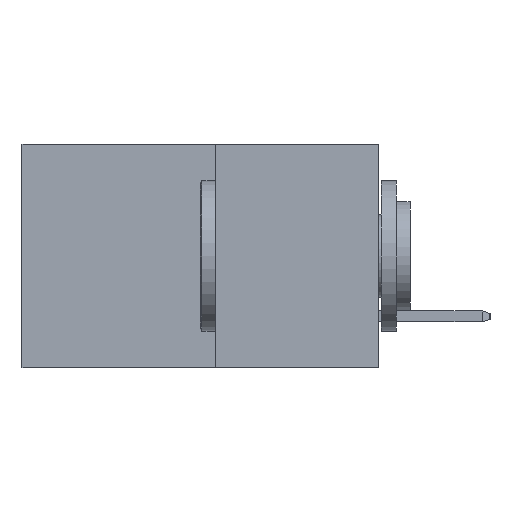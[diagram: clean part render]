
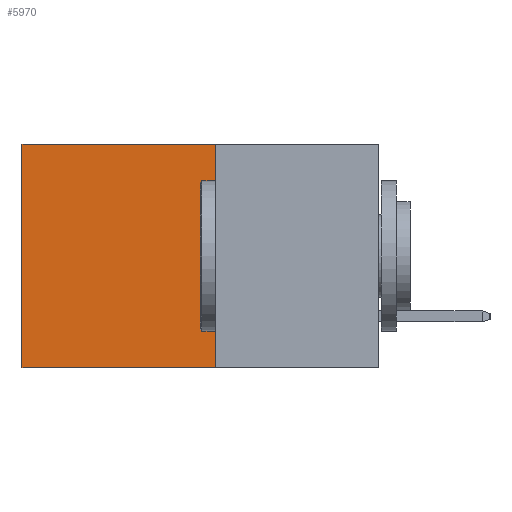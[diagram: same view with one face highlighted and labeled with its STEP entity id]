
A CAD part, left-side view. The second image highlights one B-rep face of the part: STEP entity #5970.
In plain terms, the highlighted planar face has unit normal (-1, 0, 0).
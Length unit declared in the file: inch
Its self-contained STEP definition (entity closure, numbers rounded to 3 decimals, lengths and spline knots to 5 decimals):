
#298 = VERTEX_POINT ( 'NONE', #609 ) ;
#563 = VERTEX_POINT ( 'NONE', #2316 ) ;
#609 = CARTESIAN_POINT ( 'NONE',  ( 0.277, 0.59, -0.37 ) ) ;
#874 = EDGE_CURVE ( 'NONE', #563, #6993, #4455, .T. ) ;
#967 = DIRECTION ( 'NONE',  ( 0., 0., -1. ) ) ;
#1221 = DIRECTION ( 'NONE',  ( 0., 0., -1. ) ) ;
#1283 = DIRECTION ( 'NONE',  ( 1., 0., 0. ) ) ;
#1301 = PLANE ( 'NONE',  #3410 ) ;
#1597 = CARTESIAN_POINT ( 'NONE',  ( 0.277, 0.27, -0.37 ) ) ;
#1665 = ORIENTED_EDGE ( 'NONE', *, *, #874, .T. ) ;
#1707 = EDGE_CURVE ( 'NONE', #6993, #298, #10107, .T. ) ;
#1984 = CARTESIAN_POINT ( 'NONE',  ( 0.277, 0.27, -0.37 ) ) ;
#2118 = VECTOR ( 'NONE', #3035, 39.37008 ) ;
#2316 = CARTESIAN_POINT ( 'NONE',  ( 0.277, 0.27, 0. ) ) ;
#2654 = VERTEX_POINT ( 'NONE', #1984 ) ;
#2937 = VECTOR ( 'NONE', #967, 39.37008 ) ;
#3006 = EDGE_CURVE ( 'NONE', #563, #2654, #6020, .T. ) ;
#3013 = CARTESIAN_POINT ( 'NONE',  ( 0.277, 0.59, -0.37 ) ) ;
#3035 = DIRECTION ( 'NONE',  ( 0., 1., 0. ) ) ;
#3410 = AXIS2_PLACEMENT_3D ( 'NONE', #1597, #1283, #1221 ) ;
#4241 = ORIENTED_EDGE ( 'NONE', *, *, #6172, .F. ) ;
#4455 = LINE ( 'NONE', #10359, #2118 ) ;
#5346 = ORIENTED_EDGE ( 'NONE', *, *, #1707, .T. ) ;
#5587 = ORIENTED_EDGE ( 'NONE', *, *, #3006, .F. ) ;
#5970 = ADVANCED_FACE ( 'NONE', ( #9192 ), #1301, .F. ) ;
#6020 = LINE ( 'NONE', #10955, #10348 ) ;
#6172 = EDGE_CURVE ( 'NONE', #2654, #298, #7043, .T. ) ;
#6993 = VERTEX_POINT ( 'NONE', #9894 ) ;
#7043 = LINE ( 'NONE', #9688, #11332 ) ;
#8828 = DIRECTION ( 'NONE',  ( 0., 1., 0. ) ) ;
#9192 = FACE_OUTER_BOUND ( 'NONE', #10472, .T. ) ;
#9688 = CARTESIAN_POINT ( 'NONE',  ( 0.277, 0.27, -0.37 ) ) ;
#9894 = CARTESIAN_POINT ( 'NONE',  ( 0.277, 0.59, 0. ) ) ;
#10107 = LINE ( 'NONE', #3013, #2937 ) ;
#10348 = VECTOR ( 'NONE', #11165, 39.37008 ) ;
#10359 = CARTESIAN_POINT ( 'NONE',  ( 0.277, 0.27, 0. ) ) ;
#10472 = EDGE_LOOP ( 'NONE', ( #5346, #4241, #5587, #1665 ) ) ;
#10955 = CARTESIAN_POINT ( 'NONE',  ( 0.277, 0.27, -0.37 ) ) ;
#11165 = DIRECTION ( 'NONE',  ( 0., 0., -1. ) ) ;
#11332 = VECTOR ( 'NONE', #8828, 39.37008 ) ;
